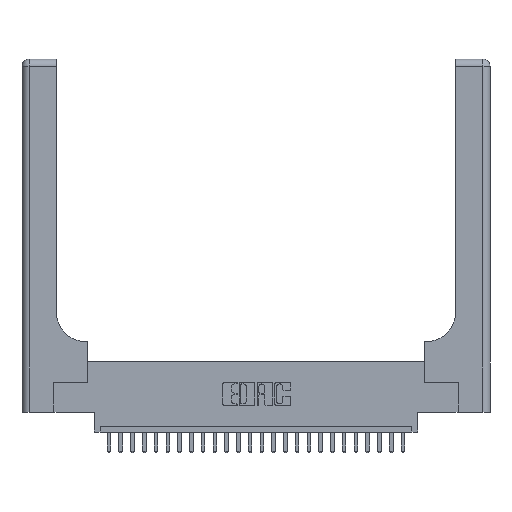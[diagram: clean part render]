
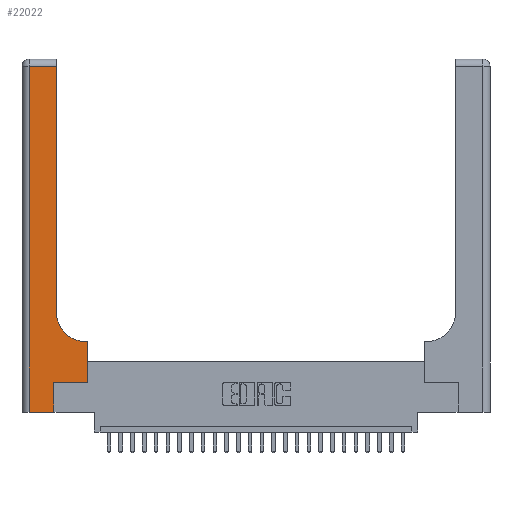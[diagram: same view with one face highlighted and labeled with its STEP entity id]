
A CAD part, top view. The second image highlights one B-rep face of the part: STEP entity #22022.
In plain terms, the highlighted planar face has unit normal (0, 0, 1).
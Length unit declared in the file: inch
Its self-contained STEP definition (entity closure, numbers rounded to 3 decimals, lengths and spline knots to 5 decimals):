
#432 = CARTESIAN_POINT ( 'NONE',  ( 0.5415, 0.85, 0.37 ) ) ;
#832 = VECTOR ( 'NONE', #19692, 39.37008 ) ;
#920 = EDGE_LOOP ( 'NONE', ( #18286, #18190, #10644, #15852, #5921, #20341, #3286, #23512, #18538 ) ) ;
#1647 = FACE_OUTER_BOUND ( 'NONE', #920, .T. ) ;
#2597 = EDGE_CURVE ( 'NONE', #6240, #13618, #4401, .T. ) ;
#2649 = EDGE_CURVE ( 'NONE', #6195, #7469, #9310, .T. ) ;
#3052 = VECTOR ( 'NONE', #13378, 39.37008 ) ;
#3080 = VECTOR ( 'NONE', #5090, 39.37008 ) ;
#3286 = ORIENTED_EDGE ( 'NONE', *, *, #20273, .T. ) ;
#3743 = DIRECTION ( 'NONE',  ( -1., 0., 0. ) ) ;
#4401 = LINE ( 'NONE', #23207, #26049 ) ;
#4599 = EDGE_CURVE ( 'NONE', #11243, #6195, #9854, .T. ) ;
#4643 = CARTESIAN_POINT ( 'NONE',  ( 0.06, 3., 0.37 ) ) ;
#5090 = DIRECTION ( 'NONE',  ( 0., 1., 0. ) ) ;
#5655 = CARTESIAN_POINT ( 'NONE',  ( 0., 2.94, 0.37 ) ) ;
#5707 = DIRECTION ( 'NONE',  ( 0., 1., 0. ) ) ;
#5921 = ORIENTED_EDGE ( 'NONE', *, *, #12658, .T. ) ;
#6195 = VERTEX_POINT ( 'NONE', #21238 ) ;
#6240 = VERTEX_POINT ( 'NONE', #19321 ) ;
#6303 = EDGE_CURVE ( 'NONE', #20016, #11243, #23526, .T. ) ;
#6509 = DIRECTION ( 'NONE',  ( 1., 0., 0. ) ) ;
#6510 = VECTOR ( 'NONE', #20117, 39.37008 ) ;
#7469 = VERTEX_POINT ( 'NONE', #24452 ) ;
#7615 = VERTEX_POINT ( 'NONE', #22345 ) ;
#7633 = AXIS2_PLACEMENT_3D ( 'NONE', #432, #8945, #6509 ) ;
#8122 = EDGE_CURVE ( 'NONE', #9219, #8960, #13020, .T. ) ;
#8945 = DIRECTION ( 'NONE',  ( 0., 0., -1. ) ) ;
#8960 = VERTEX_POINT ( 'NONE', #20345 ) ;
#9182 = CARTESIAN_POINT ( 'NONE',  ( 0., 0., 0.37 ) ) ;
#9219 = VERTEX_POINT ( 'NONE', #25703 ) ;
#9310 = LINE ( 'NONE', #9182, #3052 ) ;
#9733 = VECTOR ( 'NONE', #5707, 39.37008 ) ;
#9854 = LINE ( 'NONE', #4643, #24948 ) ;
#10292 = CARTESIAN_POINT ( 'NONE',  ( 0.5585, 0.25, 0.37 ) ) ;
#10644 = ORIENTED_EDGE ( 'NONE', *, *, #4599, .T. ) ;
#10649 = CARTESIAN_POINT ( 'NONE',  ( 0.269, 0., 0.37 ) ) ;
#11243 = VERTEX_POINT ( 'NONE', #13507 ) ;
#12021 = LINE ( 'NONE', #10649, #832 ) ;
#12658 = EDGE_CURVE ( 'NONE', #7469, #6240, #12021, .T. ) ;
#13020 = LINE ( 'NONE', #16096, #18535 ) ;
#13378 = DIRECTION ( 'NONE',  ( 1., 0., 0. ) ) ;
#13507 = CARTESIAN_POINT ( 'NONE',  ( 0.06, 2.94, 0.37 ) ) ;
#13618 = VERTEX_POINT ( 'NONE', #10292 ) ;
#13811 = EDGE_CURVE ( 'NONE', #7615, #20016, #20800, .T. ) ;
#14059 = PLANE ( 'NONE',  #25133 ) ;
#15852 = ORIENTED_EDGE ( 'NONE', *, *, #2649, .T. ) ;
#16096 = CARTESIAN_POINT ( 'NONE',  ( 0.2915, 0.6, 0.37 ) ) ;
#17459 = CARTESIAN_POINT ( 'NONE',  ( 0.2915, 3., 0.37 ) ) ;
#18135 = EDGE_CURVE ( 'NONE', #8960, #7615, #20280, .T. ) ;
#18190 = ORIENTED_EDGE ( 'NONE', *, *, #6303, .T. ) ;
#18286 = ORIENTED_EDGE ( 'NONE', *, *, #13811, .T. ) ;
#18535 = VECTOR ( 'NONE', #20669, 39.37008 ) ;
#18538 = ORIENTED_EDGE ( 'NONE', *, *, #18135, .T. ) ;
#18901 = DIRECTION ( 'NONE',  ( 1., 0., 0. ) ) ;
#19108 = CARTESIAN_POINT ( 'NONE',  ( 0.2915, 2.94, 0.37 ) ) ;
#19321 = CARTESIAN_POINT ( 'NONE',  ( 0.269, 0.25, 0.37 ) ) ;
#19564 = LINE ( 'NONE', #26687, #9733 ) ;
#19692 = DIRECTION ( 'NONE',  ( 0., 1., 0. ) ) ;
#20016 = VERTEX_POINT ( 'NONE', #19108 ) ;
#20117 = DIRECTION ( 'NONE',  ( -1., 0., 0. ) ) ;
#20273 = EDGE_CURVE ( 'NONE', #13618, #9219, #19564, .T. ) ;
#20280 = CIRCLE ( 'NONE', #7633, 0.25 ) ;
#20341 = ORIENTED_EDGE ( 'NONE', *, *, #2597, .T. ) ;
#20345 = CARTESIAN_POINT ( 'NONE',  ( 0.5415, 0.6, 0.37 ) ) ;
#20669 = DIRECTION ( 'NONE',  ( -1., 0., 0. ) ) ;
#20800 = LINE ( 'NONE', #17459, #3080 ) ;
#21238 = CARTESIAN_POINT ( 'NONE',  ( 0.06, 0., 0.37 ) ) ;
#22022 = ADVANCED_FACE ( 'NONE', ( #1647 ), #14059, .F. ) ;
#22345 = CARTESIAN_POINT ( 'NONE',  ( 0.2915, 0.85, 0.37 ) ) ;
#22636 = CARTESIAN_POINT ( 'NONE',  ( 0., 3., 0.37 ) ) ;
#23207 = CARTESIAN_POINT ( 'NONE',  ( 0.269, 0.25, 0.37 ) ) ;
#23512 = ORIENTED_EDGE ( 'NONE', *, *, #8122, .T. ) ;
#23526 = LINE ( 'NONE', #5655, #6510 ) ;
#23698 = DIRECTION ( 'NONE',  ( 0., -1., 0. ) ) ;
#24452 = CARTESIAN_POINT ( 'NONE',  ( 0.269, 0., 0.37 ) ) ;
#24479 = DIRECTION ( 'NONE',  ( 0., 0., -1. ) ) ;
#24948 = VECTOR ( 'NONE', #23698, 39.37008 ) ;
#25133 = AXIS2_PLACEMENT_3D ( 'NONE', #22636, #24479, #3743 ) ;
#25703 = CARTESIAN_POINT ( 'NONE',  ( 0.5585, 0.6, 0.37 ) ) ;
#26049 = VECTOR ( 'NONE', #18901, 39.37008 ) ;
#26687 = CARTESIAN_POINT ( 'NONE',  ( 0.5585, 0.25, 0.37 ) ) ;
